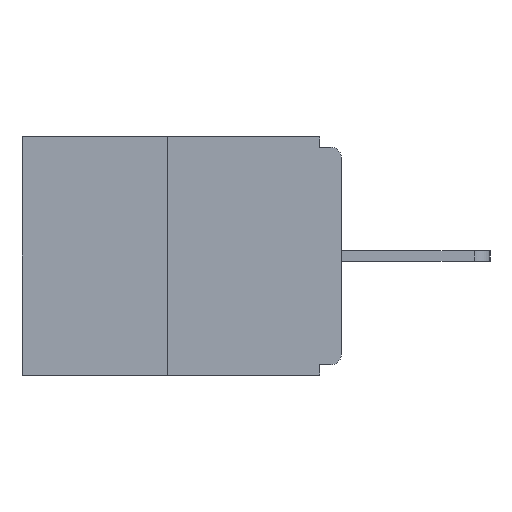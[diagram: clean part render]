
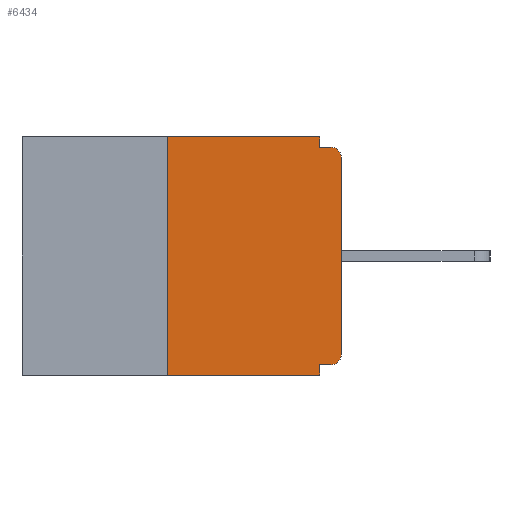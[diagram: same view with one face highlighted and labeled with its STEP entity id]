
A CAD part, left-side view. The second image highlights one B-rep face of the part: STEP entity #6434.
In plain terms, the highlighted planar face has unit normal (-1, 0, 0).
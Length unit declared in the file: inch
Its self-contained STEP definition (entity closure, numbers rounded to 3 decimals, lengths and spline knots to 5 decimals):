
#949 = CARTESIAN_POINT ( 'NONE',  ( 0., 0.031, 0. ) ) ;
#1065 = DIRECTION ( 'NONE',  ( 0., 0., -1. ) ) ;
#1472 = LINE ( 'NONE', #1679, #8357 ) ;
#1679 = CARTESIAN_POINT ( 'NONE',  ( 0., 0.031, -0.343 ) ) ;
#2086 = CIRCLE ( 'NONE', #18754, 0.015 ) ;
#2202 = VERTEX_POINT ( 'NONE', #2657 ) ;
#2657 = CARTESIAN_POINT ( 'NONE',  ( 0., 0.015, -0.328 ) ) ;
#2792 = ORIENTED_EDGE ( 'NONE', *, *, #5923, .F. ) ;
#3136 = DIRECTION ( 'NONE',  ( -1., 0., 0. ) ) ;
#4033 = ORIENTED_EDGE ( 'NONE', *, *, #15957, .F. ) ;
#4515 = CARTESIAN_POINT ( 'NONE',  ( 0., 0.46, 0. ) ) ;
#4575 = VECTOR ( 'NONE', #9042, 39.37008 ) ;
#4601 = LINE ( 'NONE', #18907, #13457 ) ;
#4758 = VECTOR ( 'NONE', #4863, 39.37008 ) ;
#4863 = DIRECTION ( 'NONE',  ( 0., -1., 0. ) ) ;
#4872 = ORIENTED_EDGE ( 'NONE', *, *, #8327, .T. ) ;
#4909 = DIRECTION ( 'NONE',  ( 0., 0., 1. ) ) ;
#5167 = EDGE_CURVE ( 'NONE', #8918, #15984, #2086, .T. ) ;
#5368 = EDGE_CURVE ( 'NONE', #8486, #5690, #14596, .T. ) ;
#5570 = VERTEX_POINT ( 'NONE', #5828 ) ;
#5690 = VERTEX_POINT ( 'NONE', #11175 ) ;
#5754 = PLANE ( 'NONE',  #16352 ) ;
#5828 = CARTESIAN_POINT ( 'NONE',  ( 0., 0.031, -0.015 ) ) ;
#5923 = EDGE_CURVE ( 'NONE', #2202, #11414, #11372, .T. ) ;
#6434 = ADVANCED_FACE ( 'NONE', ( #9105 ), #5754, .F. ) ;
#6658 = ORIENTED_EDGE ( 'NONE', *, *, #8635, .F. ) ;
#6673 = VERTEX_POINT ( 'NONE', #20474 ) ;
#6684 = EDGE_CURVE ( 'NONE', #11414, #6673, #1472, .T. ) ;
#7615 = DIRECTION ( 'NONE',  ( 0., -1., 0. ) ) ;
#7751 = CARTESIAN_POINT ( 'NONE',  ( 0., 0., 0. ) ) ;
#7835 = EDGE_CURVE ( 'NONE', #9626, #8918, #12488, .T. ) ;
#8025 = DIRECTION ( 'NONE',  ( 0., 0., -1. ) ) ;
#8082 = VECTOR ( 'NONE', #16552, 39.37008 ) ;
#8205 = VECTOR ( 'NONE', #19598, 39.37008 ) ;
#8327 = EDGE_CURVE ( 'NONE', #2202, #9626, #18408, .T. ) ;
#8357 = VECTOR ( 'NONE', #8025, 39.37008 ) ;
#8486 = VERTEX_POINT ( 'NONE', #11695 ) ;
#8635 = EDGE_CURVE ( 'NONE', #5690, #13884, #19055, .T. ) ;
#8667 = ORIENTED_EDGE ( 'NONE', *, *, #5167, .T. ) ;
#8918 = VERTEX_POINT ( 'NONE', #15285 ) ;
#9042 = DIRECTION ( 'NONE',  ( 0., 0., -1. ) ) ;
#9105 = FACE_OUTER_BOUND ( 'NONE', #10128, .T. ) ;
#9158 = CARTESIAN_POINT ( 'NONE',  ( 0., 0., -0.313 ) ) ;
#9256 = LINE ( 'NONE', #18646, #4575 ) ;
#9425 = AXIS2_PLACEMENT_3D ( 'NONE', #14168, #3136, #11071 ) ;
#9489 = VECTOR ( 'NONE', #4909, 39.37008 ) ;
#9626 = VERTEX_POINT ( 'NONE', #9158 ) ;
#10128 = EDGE_LOOP ( 'NONE', ( #6658, #10341, #12666, #13009, #2792, #4872, #17321, #8667, #18498, #4033 ) ) ;
#10341 = ORIENTED_EDGE ( 'NONE', *, *, #5368, .F. ) ;
#11046 = CARTESIAN_POINT ( 'NONE',  ( 0., 0.46, 0. ) ) ;
#11071 = DIRECTION ( 'NONE',  ( 0., 0., -1. ) ) ;
#11175 = CARTESIAN_POINT ( 'NONE',  ( 0., 0.25, 0. ) ) ;
#11372 = LINE ( 'NONE', #13021, #8205 ) ;
#11414 = VERTEX_POINT ( 'NONE', #19441 ) ;
#11695 = CARTESIAN_POINT ( 'NONE',  ( 0., 0.25, -0.343 ) ) ;
#12488 = LINE ( 'NONE', #7751, #14703 ) ;
#12666 = ORIENTED_EDGE ( 'NONE', *, *, #19220, .T. ) ;
#13009 = ORIENTED_EDGE ( 'NONE', *, *, #6684, .F. ) ;
#13021 = CARTESIAN_POINT ( 'NONE',  ( 0., 0., -0.328 ) ) ;
#13457 = VECTOR ( 'NONE', #7615, 39.37008 ) ;
#13731 = CARTESIAN_POINT ( 'NONE',  ( 0., 0.015, -0.015 ) ) ;
#13884 = VERTEX_POINT ( 'NONE', #949 ) ;
#14168 = CARTESIAN_POINT ( 'NONE',  ( 0., 0.015, -0.313 ) ) ;
#14596 = LINE ( 'NONE', #15882, #9489 ) ;
#14703 = VECTOR ( 'NONE', #17159, 39.37008 ) ;
#15285 = CARTESIAN_POINT ( 'NONE',  ( 0., 0., -0.03 ) ) ;
#15662 = DIRECTION ( 'NONE',  ( 0., 0., -1. ) ) ;
#15775 = DIRECTION ( 'NONE',  ( -1., 0., 0. ) ) ;
#15882 = CARTESIAN_POINT ( 'NONE',  ( 0., 0.25, 0. ) ) ;
#15957 = EDGE_CURVE ( 'NONE', #13884, #5570, #9256, .T. ) ;
#15984 = VERTEX_POINT ( 'NONE', #13731 ) ;
#16352 = AXIS2_PLACEMENT_3D ( 'NONE', #4515, #20371, #1065 ) ;
#16552 = DIRECTION ( 'NONE',  ( 0., -1., 0. ) ) ;
#17159 = DIRECTION ( 'NONE',  ( 0., 0., 1. ) ) ;
#17321 = ORIENTED_EDGE ( 'NONE', *, *, #7835, .T. ) ;
#17899 = CARTESIAN_POINT ( 'NONE',  ( 0., 0.46, -0.343 ) ) ;
#18408 = CIRCLE ( 'NONE', #9425, 0.015 ) ;
#18498 = ORIENTED_EDGE ( 'NONE', *, *, #20359, .F. ) ;
#18646 = CARTESIAN_POINT ( 'NONE',  ( 0., 0.031, 0. ) ) ;
#18754 = AXIS2_PLACEMENT_3D ( 'NONE', #20572, #15775, #15662 ) ;
#18907 = CARTESIAN_POINT ( 'NONE',  ( 0., 0., -0.015 ) ) ;
#19055 = LINE ( 'NONE', #11046, #4758 ) ;
#19220 = EDGE_CURVE ( 'NONE', #8486, #6673, #19583, .T. ) ;
#19441 = CARTESIAN_POINT ( 'NONE',  ( 0., 0.031, -0.328 ) ) ;
#19583 = LINE ( 'NONE', #17899, #8082 ) ;
#19598 = DIRECTION ( 'NONE',  ( 0., 1., 0. ) ) ;
#20359 = EDGE_CURVE ( 'NONE', #5570, #15984, #4601, .T. ) ;
#20371 = DIRECTION ( 'NONE',  ( 1., 0., 0. ) ) ;
#20474 = CARTESIAN_POINT ( 'NONE',  ( 0., 0.031, -0.343 ) ) ;
#20572 = CARTESIAN_POINT ( 'NONE',  ( 0., 0.015, -0.03 ) ) ;
